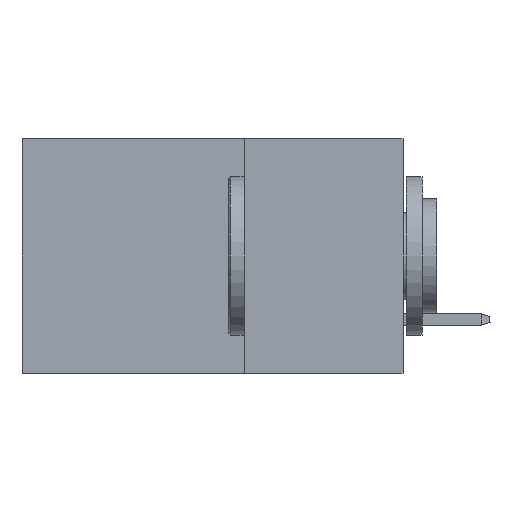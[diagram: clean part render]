
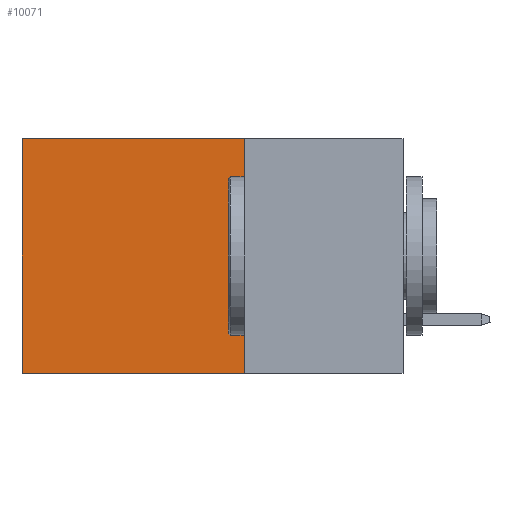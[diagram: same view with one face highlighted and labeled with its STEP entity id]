
A CAD part, left-side view. The second image highlights one B-rep face of the part: STEP entity #10071.
In plain terms, the highlighted planar face has unit normal (-1, 0, 0).
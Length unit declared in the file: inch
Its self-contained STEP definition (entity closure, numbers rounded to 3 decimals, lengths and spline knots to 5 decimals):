
#245 = CARTESIAN_POINT ( 'NONE',  ( 0.2875, 0.25, 0. ) ) ;
#329 = DIRECTION ( 'NONE',  ( 0., 1., 0. ) ) ;
#1356 = CARTESIAN_POINT ( 'NONE',  ( 0.2875, 0.25, 0. ) ) ;
#2236 = EDGE_CURVE ( 'NONE', #20835, #19530, #20549, .T. ) ;
#2277 = CARTESIAN_POINT ( 'NONE',  ( 0.2875, 0.6, -0.37 ) ) ;
#2680 = CARTESIAN_POINT ( 'NONE',  ( 0.2875, 0.25, 0. ) ) ;
#3023 = VECTOR ( 'NONE', #9845, 39.37008 ) ;
#3962 = EDGE_LOOP ( 'NONE', ( #23015, #17471, #8706, #8276 ) ) ;
#5564 = DIRECTION ( 'NONE',  ( 1., 0., 0. ) ) ;
#6690 = CARTESIAN_POINT ( 'NONE',  ( 0.2875, 0.25, -0.37 ) ) ;
#6928 = AXIS2_PLACEMENT_3D ( 'NONE', #19893, #5564, #12737 ) ;
#7757 = VERTEX_POINT ( 'NONE', #2277 ) ;
#8276 = ORIENTED_EDGE ( 'NONE', *, *, #16957, .T. ) ;
#8706 = ORIENTED_EDGE ( 'NONE', *, *, #2236, .F. ) ;
#9254 = CARTESIAN_POINT ( 'NONE',  ( 0.2875, 0.6, 0. ) ) ;
#9845 = DIRECTION ( 'NONE',  ( 0., 0., -1. ) ) ;
#10071 = ADVANCED_FACE ( 'NONE', ( #14449 ), #21528, .F. ) ;
#10106 = VECTOR ( 'NONE', #329, 39.37008 ) ;
#10118 = EDGE_CURVE ( 'NONE', #19530, #7757, #19195, .T. ) ;
#10762 = VECTOR ( 'NONE', #16389, 39.37008 ) ;
#11969 = EDGE_CURVE ( 'NONE', #12245, #7757, #18112, .T. ) ;
#12245 = VERTEX_POINT ( 'NONE', #16368 ) ;
#12585 = VECTOR ( 'NONE', #17068, 39.37008 ) ;
#12737 = DIRECTION ( 'NONE',  ( 0., 0., -1. ) ) ;
#14449 = FACE_OUTER_BOUND ( 'NONE', #3962, .T. ) ;
#16368 = CARTESIAN_POINT ( 'NONE',  ( 0.2875, 0.6, 0. ) ) ;
#16389 = DIRECTION ( 'NONE',  ( 0., 0., -1. ) ) ;
#16957 = EDGE_CURVE ( 'NONE', #20835, #12245, #18805, .T. ) ;
#17068 = DIRECTION ( 'NONE',  ( 0., 1., 0. ) ) ;
#17471 = ORIENTED_EDGE ( 'NONE', *, *, #10118, .F. ) ;
#17730 = CARTESIAN_POINT ( 'NONE',  ( 0.2875, 0.25, -0.37 ) ) ;
#18112 = LINE ( 'NONE', #9254, #10762 ) ;
#18805 = LINE ( 'NONE', #1356, #10106 ) ;
#19195 = LINE ( 'NONE', #6690, #12585 ) ;
#19530 = VERTEX_POINT ( 'NONE', #17730 ) ;
#19893 = CARTESIAN_POINT ( 'NONE',  ( 0.2875, 0.25, 0. ) ) ;
#20549 = LINE ( 'NONE', #2680, #3023 ) ;
#20835 = VERTEX_POINT ( 'NONE', #245 ) ;
#21528 = PLANE ( 'NONE',  #6928 ) ;
#23015 = ORIENTED_EDGE ( 'NONE', *, *, #11969, .T. ) ;
